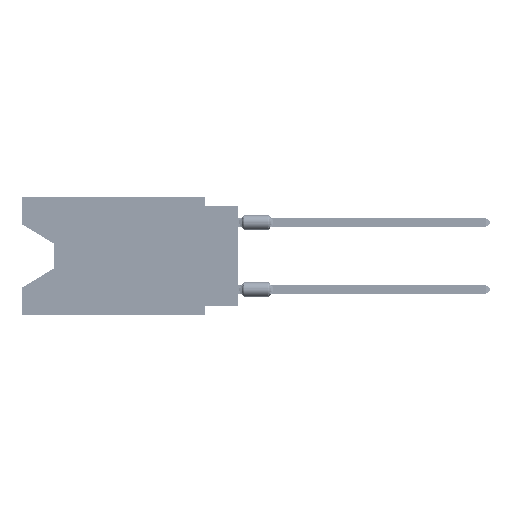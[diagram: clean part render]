
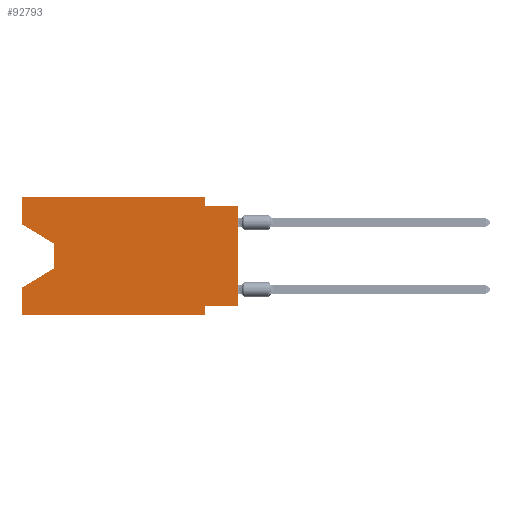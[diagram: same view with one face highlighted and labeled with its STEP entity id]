
A CAD part, left-side view. The second image highlights one B-rep face of the part: STEP entity #92793.
In plain terms, the highlighted planar face has unit normal (-1, 0, 0).
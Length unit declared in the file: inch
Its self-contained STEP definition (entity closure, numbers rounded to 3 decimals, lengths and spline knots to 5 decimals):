
#2495 = LINE ( 'NONE', #57412, #112025 ) ;
#4131 = LINE ( 'NONE', #12320, #39507 ) ;
#4336 = VECTOR ( 'NONE', #28112, 39.37008 ) ;
#4865 = ORIENTED_EDGE ( 'NONE', *, *, #20785, .F. ) ;
#7762 = DIRECTION ( 'NONE',  ( 0., 0., -1. ) ) ;
#9487 = EDGE_CURVE ( 'NONE', #20087, #94699, #31567, .T. ) ;
#9551 = VERTEX_POINT ( 'NONE', #83062 ) ;
#9686 = ORIENTED_EDGE ( 'NONE', *, *, #21777, .T. ) ;
#10592 = ORIENTED_EDGE ( 'NONE', *, *, #78079, .T. ) ;
#11140 = CARTESIAN_POINT ( 'NONE',  ( 0., 0.645, -0.08025 ) ) ;
#11796 = VECTOR ( 'NONE', #23336, 39.37008 ) ;
#12320 = CARTESIAN_POINT ( 'NONE',  ( 0., 0., -0.325 ) ) ;
#12359 = ORIENTED_EDGE ( 'NONE', *, *, #14995, .F. ) ;
#13364 = CARTESIAN_POINT ( 'NONE',  ( 0., 0.55, -0.138 ) ) ;
#13532 = LINE ( 'NONE', #112356, #39197 ) ;
#13803 = VECTOR ( 'NONE', #79124, 39.37008 ) ;
#14995 = EDGE_CURVE ( 'NONE', #60998, #20087, #4131, .T. ) ;
#16574 = CARTESIAN_POINT ( 'NONE',  ( 0., 0.55, -0.138 ) ) ;
#17122 = VECTOR ( 'NONE', #30401, 39.37008 ) ;
#20087 = VERTEX_POINT ( 'NONE', #110051 ) ;
#20495 = LINE ( 'NONE', #11140, #4336 ) ;
#20785 = EDGE_CURVE ( 'NONE', #29100, #78351, #104933, .T. ) ;
#21621 = LINE ( 'NONE', #58406, #11796 ) ;
#21777 = EDGE_CURVE ( 'NONE', #60998, #78351, #26526, .T. ) ;
#23073 = LINE ( 'NONE', #24774, #56543 ) ;
#23195 = CARTESIAN_POINT ( 'NONE',  ( 0., 0.645, -0.35 ) ) ;
#23336 = DIRECTION ( 'NONE',  ( 0., 0., 1. ) ) ;
#24774 = CARTESIAN_POINT ( 'NONE',  ( 0., 0.1, 0. ) ) ;
#25917 = LINE ( 'NONE', #16574, #13803 ) ;
#26526 = LINE ( 'NONE', #70391, #64031 ) ;
#28112 = DIRECTION ( 'NONE',  ( 0., -0.855, -0.519 ) ) ;
#29100 = VERTEX_POINT ( 'NONE', #65095 ) ;
#29636 = DIRECTION ( 'NONE',  ( 0., -1., 0. ) ) ;
#30401 = DIRECTION ( 'NONE',  ( 0., 0., -1. ) ) ;
#31567 = LINE ( 'NONE', #66054, #17122 ) ;
#31841 = DIRECTION ( 'NONE',  ( 0., 0., -1. ) ) ;
#32463 = DIRECTION ( 'NONE',  ( 0., -1., 0. ) ) ;
#32939 = CARTESIAN_POINT ( 'NONE',  ( 0., 0.645, 0. ) ) ;
#35134 = ORIENTED_EDGE ( 'NONE', *, *, #82984, .F. ) ;
#35487 = ORIENTED_EDGE ( 'NONE', *, *, #83553, .F. ) ;
#36512 = AXIS2_PLACEMENT_3D ( 'NONE', #32939, #52204, #7762 ) ;
#36957 = VECTOR ( 'NONE', #29636, 39.37008 ) ;
#38001 = VECTOR ( 'NONE', #87235, 39.37008 ) ;
#38118 = DIRECTION ( 'NONE',  ( 0., 0., 1. ) ) ;
#38588 = VECTOR ( 'NONE', #32463, 39.37008 ) ;
#39197 = VECTOR ( 'NONE', #77247, 39.37008 ) ;
#39374 = ORIENTED_EDGE ( 'NONE', *, *, #53799, .T. ) ;
#39507 = VECTOR ( 'NONE', #91303, 39.37008 ) ;
#40632 = VERTEX_POINT ( 'NONE', #59650 ) ;
#40963 = ORIENTED_EDGE ( 'NONE', *, *, #114291, .T. ) ;
#43794 = CARTESIAN_POINT ( 'NONE',  ( 0., 0.645, 0. ) ) ;
#52204 = DIRECTION ( 'NONE',  ( 1., 0., 0. ) ) ;
#52539 = VERTEX_POINT ( 'NONE', #43794 ) ;
#53799 = EDGE_CURVE ( 'NONE', #95795, #72844, #20495, .T. ) ;
#56543 = VECTOR ( 'NONE', #31841, 39.37008 ) ;
#57412 = CARTESIAN_POINT ( 'NONE',  ( 0., 0.645, 0. ) ) ;
#58406 = CARTESIAN_POINT ( 'NONE',  ( 0., 0.645, 0. ) ) ;
#59650 = CARTESIAN_POINT ( 'NONE',  ( 0., 0.1, 0. ) ) ;
#60998 = VERTEX_POINT ( 'NONE', #108213 ) ;
#61476 = CARTESIAN_POINT ( 'NONE',  ( 0., 0.645, 0. ) ) ;
#64031 = VECTOR ( 'NONE', #97874, 39.37008 ) ;
#65095 = CARTESIAN_POINT ( 'NONE',  ( 0., 0.1, -0.025 ) ) ;
#66054 = CARTESIAN_POINT ( 'NONE',  ( 0., 0.1, -0.35 ) ) ;
#68198 = CARTESIAN_POINT ( 'NONE',  ( 0., 0.55, -0.212 ) ) ;
#69192 = CARTESIAN_POINT ( 'NONE',  ( 0., 0.645, -0.08025 ) ) ;
#69270 = ORIENTED_EDGE ( 'NONE', *, *, #77945, .F. ) ;
#70391 = CARTESIAN_POINT ( 'NONE',  ( 0., 0., 0. ) ) ;
#71446 = ORIENTED_EDGE ( 'NONE', *, *, #9487, .F. ) ;
#72519 = CARTESIAN_POINT ( 'NONE',  ( 0., 0., -0.025 ) ) ;
#72844 = VERTEX_POINT ( 'NONE', #13364 ) ;
#75444 = EDGE_CURVE ( 'NONE', #95795, #52539, #21621, .T. ) ;
#77247 = DIRECTION ( 'NONE',  ( 0., 0.855, -0.519 ) ) ;
#77945 = EDGE_CURVE ( 'NONE', #78849, #9551, #2495, .T. ) ;
#78079 = EDGE_CURVE ( 'NONE', #90711, #9551, #13532, .T. ) ;
#78351 = VERTEX_POINT ( 'NONE', #72519 ) ;
#78849 = VERTEX_POINT ( 'NONE', #23195 ) ;
#79124 = DIRECTION ( 'NONE',  ( 0., 0., -1. ) ) ;
#82984 = EDGE_CURVE ( 'NONE', #40632, #29100, #23073, .T. ) ;
#83062 = CARTESIAN_POINT ( 'NONE',  ( 0., 0.645, -0.26975 ) ) ;
#83454 = FACE_OUTER_BOUND ( 'NONE', #90105, .T. ) ;
#83553 = EDGE_CURVE ( 'NONE', #52539, #40632, #96573, .T. ) ;
#84574 = CARTESIAN_POINT ( 'NONE',  ( 0., 0.645, -0.35 ) ) ;
#87235 = DIRECTION ( 'NONE',  ( 0., -1., 0. ) ) ;
#87778 = ORIENTED_EDGE ( 'NONE', *, *, #91277, .T. ) ;
#89672 = ORIENTED_EDGE ( 'NONE', *, *, #75444, .F. ) ;
#90105 = EDGE_LOOP ( 'NONE', ( #39374, #87778, #10592, #69270, #40963, #71446, #12359, #9686, #4865, #35134, #35487, #89672 ) ) ;
#90711 = VERTEX_POINT ( 'NONE', #68198 ) ;
#91277 = EDGE_CURVE ( 'NONE', #72844, #90711, #25917, .T. ) ;
#91303 = DIRECTION ( 'NONE',  ( 0., 1., 0. ) ) ;
#92793 = ADVANCED_FACE ( 'NONE', ( #83454 ), #104288, .F. ) ;
#94699 = VERTEX_POINT ( 'NONE', #107196 ) ;
#95035 = CARTESIAN_POINT ( 'NONE',  ( 0., 0., -0.025 ) ) ;
#95795 = VERTEX_POINT ( 'NONE', #69192 ) ;
#96573 = LINE ( 'NONE', #61476, #38001 ) ;
#97874 = DIRECTION ( 'NONE',  ( 0., 0., 1. ) ) ;
#104288 = PLANE ( 'NONE',  #36512 ) ;
#104933 = LINE ( 'NONE', #95035, #38588 ) ;
#107196 = CARTESIAN_POINT ( 'NONE',  ( 0., 0.1, -0.35 ) ) ;
#108213 = CARTESIAN_POINT ( 'NONE',  ( 0., 0., -0.325 ) ) ;
#109755 = LINE ( 'NONE', #84574, #36957 ) ;
#110051 = CARTESIAN_POINT ( 'NONE',  ( 0., 0.1, -0.325 ) ) ;
#112025 = VECTOR ( 'NONE', #38118, 39.37008 ) ;
#112356 = CARTESIAN_POINT ( 'NONE',  ( 0., 0.55, -0.212 ) ) ;
#114291 = EDGE_CURVE ( 'NONE', #78849, #94699, #109755, .T. ) ;
